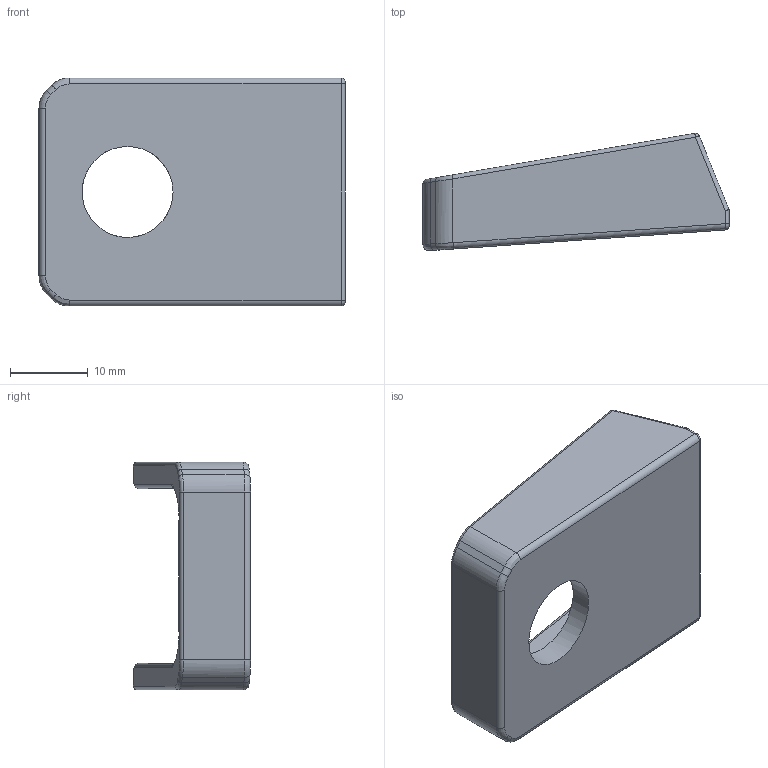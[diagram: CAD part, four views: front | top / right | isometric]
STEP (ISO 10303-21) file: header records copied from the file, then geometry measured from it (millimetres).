
FILE_DESCRIPTION(/* description */ (''),/* implementation_level */ '2;1');
FILE_NAME(/* name */ 'Baseplate - G26-G19 Angle v2.0.stp',/* time_stamp */ '2021-03-22T14:30:25-05:00',/* author */ ('johne'),/* organization */ (''),/* preprocessor_version */ 'ST-DEVELOPER v18',/* originating_system */ 'Autodesk Inventor 2020',/* authorisation */ '');
FILE_SCHEMA (('AUTOMOTIVE_DESIGN { 1 0 10303 214 3 1 1 }'));
Length unit declared in the file: inch
Products named in the file (1): Menendez Mag Baseplate v2.0
Bounding box: 39.32 x 15.04 x 29.29 mm (x, y, z)
Volume: 4548.2 mm3; surface area: 4179.3 mm2
Topology: 1 solids, 1 shells, 97 faces, 231 edges, 136 vertices
Faces by surface type: cylinder 49, bspline 20, plane 20, torus 6, sphere 2
Full cylindrical faces by diameter (mm): 11.684 x1
Entity records: 3322 total; most frequent: CARTESIAN_POINT 1041, DIRECTION 487, ORIENTED_EDGE 462, EDGE_CURVE 231, AXIS2_PLACEMENT_3D 192, VERTEX_POINT 136, LINE 103, VECTOR 103
